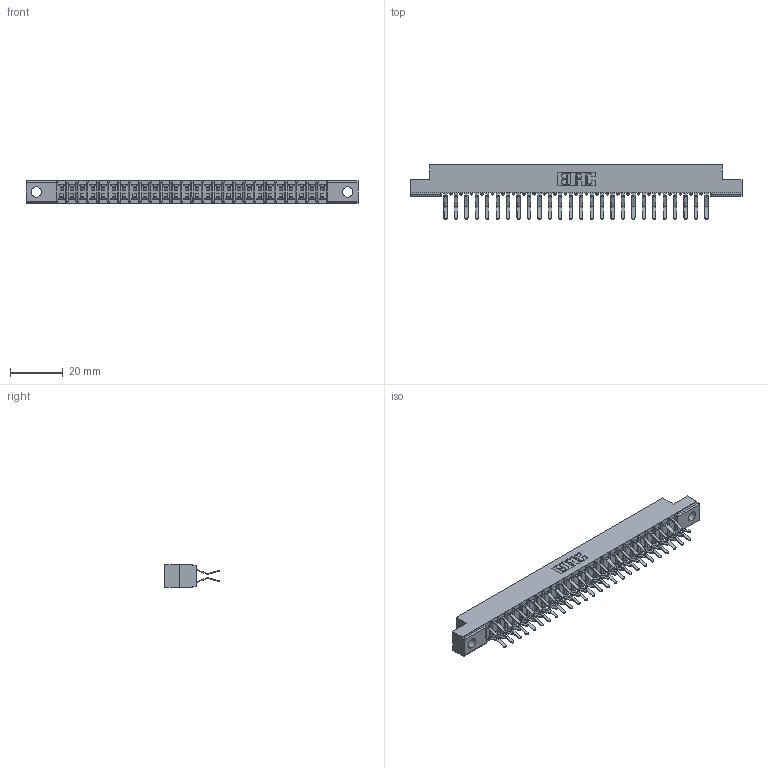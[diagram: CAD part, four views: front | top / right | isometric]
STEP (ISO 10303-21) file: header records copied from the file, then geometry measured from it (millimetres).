
FILE_DESCRIPTION (( 'STEP AP203' ), '1' );
FILE_NAME ('357-052-560-202.STEP', '2019-09-19T03:41:40', ( '' ), ( '' ), 'SwSTEP 2.0', 'SolidWorks 2016', '' );
FILE_SCHEMA (( 'CONFIG_CONTROL_DESIGN' ));
Length unit declared in the file: inch
Products named in the file (3): 357-052-560-202; 307-290-001_560; 307 Part_.128 Dia Mounting Holes
Assembly tree (53 placements, depth 2):
  357-052-560-202
    307 Part_.128 Dia Mounting Holes
    307-290-001_560  x52
Bounding box: 126.03 x 20.73 x 8.71 mm (x, y, z)
Volume: 8220.5 mm3; surface area: 14968.5 mm2
Topology: 53 solids, 53 shells, 2745 faces, 7707 edges, 4994 vertices
Faces by surface type: plane 1786, cylinder 905, sphere 54
Entity records: 25200 total; most frequent: CARTESIAN_POINT 4126, ORIENTED_EDGE 4086, DIRECTION 4049, EDGE_CURVE 2043, VECTOR 1559, LINE 1559, VERTEX_POINT 1322, AXIS2_PLACEMENT_3D 1245
